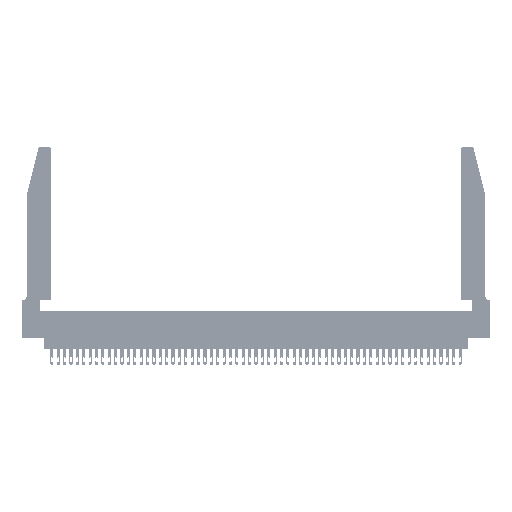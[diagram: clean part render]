
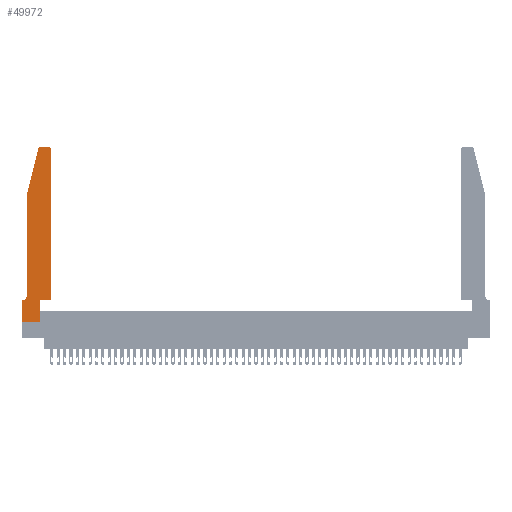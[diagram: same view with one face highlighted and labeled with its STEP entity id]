
A CAD part, top view. The second image highlights one B-rep face of the part: STEP entity #49972.
In plain terms, the highlighted planar face has unit normal (0, 0, 1).
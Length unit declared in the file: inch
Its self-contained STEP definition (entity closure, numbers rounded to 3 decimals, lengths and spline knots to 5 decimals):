
#462 = DIRECTION ( 'NONE',  ( 0., 0., 1. ) ) ;
#658 = CARTESIAN_POINT ( 'NONE',  ( 0.0755, 2., 0.37 ) ) ;
#903 = VERTEX_POINT ( 'NONE', #42194 ) ;
#2040 = CARTESIAN_POINT ( 'NONE',  ( 0.284, 2.75, 0.37 ) ) ;
#2953 = VERTEX_POINT ( 'NONE', #20163 ) ;
#4438 = CARTESIAN_POINT ( 'NONE',  ( 0.0055, 0.42, 0.37 ) ) ;
#5208 = CARTESIAN_POINT ( 'NONE',  ( 0., 0., 0.37 ) ) ;
#5640 = ORIENTED_EDGE ( 'NONE', *, *, #29134, .T. ) ;
#6308 = LINE ( 'NONE', #21184, #25427 ) ;
#6804 = CARTESIAN_POINT ( 'NONE',  ( 0., 0., 0.37 ) ) ;
#7109 = VERTEX_POINT ( 'NONE', #13375 ) ;
#8447 = ORIENTED_EDGE ( 'NONE', *, *, #38276, .T. ) ;
#8705 = DIRECTION ( 'NONE',  ( 1., 0., 0. ) ) ;
#8990 = DIRECTION ( 'NONE',  ( 1., 0., 0. ) ) ;
#9682 = CARTESIAN_POINT ( 'NONE',  ( 0., 0., 0.37 ) ) ;
#9719 = CIRCLE ( 'NONE', #34221, 0.07 ) ;
#10362 = EDGE_CURVE ( 'NONE', #13589, #39218, #52723, .T. ) ;
#10477 = ORIENTED_EDGE ( 'NONE', *, *, #38876, .T. ) ;
#10896 = EDGE_LOOP ( 'NONE', ( #40590, #37836, #21399, #5640, #10477, #12470, #46249, #42510, #8447, #43906, #12363, #19804 ) ) ;
#11210 = VECTOR ( 'NONE', #14097, 39.37008 ) ;
#11883 = EDGE_CURVE ( 'NONE', #49871, #12930, #48112, .T. ) ;
#12033 = CARTESIAN_POINT ( 'NONE',  ( 0.4505, 0.35, 0.37 ) ) ;
#12363 = ORIENTED_EDGE ( 'NONE', *, *, #52319, .T. ) ;
#12470 = ORIENTED_EDGE ( 'NONE', *, *, #20970, .T. ) ;
#12533 = CARTESIAN_POINT ( 'NONE',  ( 0.2865, 0.35, 0.37 ) ) ;
#12930 = VERTEX_POINT ( 'NONE', #16961 ) ;
#13375 = CARTESIAN_POINT ( 'NONE',  ( 0.0055, 0.35, 0.37 ) ) ;
#13589 = VERTEX_POINT ( 'NONE', #49819 ) ;
#14097 = DIRECTION ( 'NONE',  ( 1., 0., 0. ) ) ;
#14239 = LINE ( 'NONE', #9682, #48590 ) ;
#15106 = VECTOR ( 'NONE', #32308, 39.37008 ) ;
#15111 = AXIS2_PLACEMENT_3D ( 'NONE', #41087, #36807, #8705 ) ;
#15677 = DIRECTION ( 'NONE',  ( -1., 0., 0. ) ) ;
#15929 = EDGE_CURVE ( 'NONE', #2953, #44714, #44514, .T. ) ;
#16375 = LINE ( 'NONE', #12033, #15106 ) ;
#16961 = CARTESIAN_POINT ( 'NONE',  ( 0.4505, 0.35, 0.37 ) ) ;
#17741 = CARTESIAN_POINT ( 'NONE',  ( 0.2865, 0., 0.37 ) ) ;
#18474 = EDGE_CURVE ( 'NONE', #903, #32754, #14239, .T. ) ;
#18583 = CIRCLE ( 'NONE', #51100, 0.03 ) ;
#18783 = EDGE_CURVE ( 'NONE', #39218, #41170, #47335, .T. ) ;
#19001 = CARTESIAN_POINT ( 'NONE',  ( 0.4205, 2.75, 0.37 ) ) ;
#19692 = EDGE_CURVE ( 'NONE', #41170, #2953, #18583, .T. ) ;
#19804 = ORIENTED_EDGE ( 'NONE', *, *, #10362, .T. ) ;
#19895 = CARTESIAN_POINT ( 'NONE',  ( 0.2865, 0.35, 0.37 ) ) ;
#20163 = CARTESIAN_POINT ( 'NONE',  ( 0.25487, 2.72718, 0.37 ) ) ;
#20822 = DIRECTION ( 'NONE',  ( -1., 0., 0. ) ) ;
#20970 = EDGE_CURVE ( 'NONE', #7109, #903, #6308, .T. ) ;
#21184 = CARTESIAN_POINT ( 'NONE',  ( 0.0755, 0.35, 0.37 ) ) ;
#21399 = ORIENTED_EDGE ( 'NONE', *, *, #15929, .T. ) ;
#21459 = CARTESIAN_POINT ( 'NONE',  ( 0.0755, 2., 0.37 ) ) ;
#22464 = VECTOR ( 'NONE', #48908, 39.37008 ) ;
#23045 = VECTOR ( 'NONE', #29049, 39.37008 ) ;
#23786 = CARTESIAN_POINT ( 'NONE',  ( 0.0755, 2., 0.37 ) ) ;
#24588 = VERTEX_POINT ( 'NONE', #47378 ) ;
#25427 = VECTOR ( 'NONE', #41481, 39.37008 ) ;
#25846 = DIRECTION ( 'NONE',  ( 0., -1., 0. ) ) ;
#26544 = CARTESIAN_POINT ( 'NONE',  ( 0.284, 2.72, 0.37 ) ) ;
#27489 = LINE ( 'NONE', #12533, #23045 ) ;
#29049 = DIRECTION ( 'NONE',  ( 0., 1., 0. ) ) ;
#29134 = EDGE_CURVE ( 'NONE', #44714, #24588, #38420, .T. ) ;
#29282 = FACE_OUTER_BOUND ( 'NONE', #10896, .T. ) ;
#31175 = CARTESIAN_POINT ( 'NONE',  ( 0.2605, 2.75, 0.37 ) ) ;
#32308 = DIRECTION ( 'NONE',  ( 0., 1., 0. ) ) ;
#32522 = VECTOR ( 'NONE', #8990, 39.37008 ) ;
#32754 = VERTEX_POINT ( 'NONE', #6804 ) ;
#32894 = PLANE ( 'NONE',  #15111 ) ;
#33052 = DIRECTION ( 'NONE',  ( 1., 0., 0. ) ) ;
#34221 = AXIS2_PLACEMENT_3D ( 'NONE', #4438, #41127, #20822 ) ;
#36807 = DIRECTION ( 'NONE',  ( 0., 0., 1. ) ) ;
#36987 = LINE ( 'NONE', #5208, #32522 ) ;
#37033 = CARTESIAN_POINT ( 'NONE',  ( 0.4205, 2.72, 0.37 ) ) ;
#37836 = ORIENTED_EDGE ( 'NONE', *, *, #19692, .T. ) ;
#38276 = EDGE_CURVE ( 'NONE', #50341, #49871, #27489, .T. ) ;
#38420 = LINE ( 'NONE', #658, #22464 ) ;
#38485 = CARTESIAN_POINT ( 'NONE',  ( 0.4505, 0.35, 0.37 ) ) ;
#38876 = EDGE_CURVE ( 'NONE', #24588, #7109, #9719, .T. ) ;
#39218 = VERTEX_POINT ( 'NONE', #19001 ) ;
#39708 = EDGE_CURVE ( 'NONE', #32754, #50341, #36987, .T. ) ;
#40590 = ORIENTED_EDGE ( 'NONE', *, *, #18783, .T. ) ;
#41087 = CARTESIAN_POINT ( 'NONE',  ( 0., 0.35, 0.37 ) ) ;
#41127 = DIRECTION ( 'NONE',  ( 0., 0., -1. ) ) ;
#41170 = VERTEX_POINT ( 'NONE', #2040 ) ;
#41302 = DIRECTION ( 'NONE',  ( 0., 0., 1. ) ) ;
#41481 = DIRECTION ( 'NONE',  ( -1., 0., 0. ) ) ;
#42194 = CARTESIAN_POINT ( 'NONE',  ( 0., 0.35, 0.37 ) ) ;
#42510 = ORIENTED_EDGE ( 'NONE', *, *, #39708, .T. ) ;
#43906 = ORIENTED_EDGE ( 'NONE', *, *, #11883, .T. ) ;
#44514 = LINE ( 'NONE', #21459, #52178 ) ;
#44714 = VERTEX_POINT ( 'NONE', #23786 ) ;
#45031 = DIRECTION ( 'NONE',  ( 1., 0., 0. ) ) ;
#45478 = DIRECTION ( 'NONE',  ( -0.239, -0.971, 0. ) ) ;
#46058 = VECTOR ( 'NONE', #15677, 39.37008 ) ;
#46249 = ORIENTED_EDGE ( 'NONE', *, *, #18474, .T. ) ;
#47335 = LINE ( 'NONE', #31175, #46058 ) ;
#47378 = CARTESIAN_POINT ( 'NONE',  ( 0.0755, 0.42, 0.37 ) ) ;
#48112 = LINE ( 'NONE', #38485, #11210 ) ;
#48590 = VECTOR ( 'NONE', #25846, 39.37008 ) ;
#48908 = DIRECTION ( 'NONE',  ( 0., -1., 0. ) ) ;
#49819 = CARTESIAN_POINT ( 'NONE',  ( 0.4505, 2.72, 0.37 ) ) ;
#49871 = VERTEX_POINT ( 'NONE', #19895 ) ;
#49972 = ADVANCED_FACE ( 'NONE', ( #29282 ), #32894, .T. ) ;
#50341 = VERTEX_POINT ( 'NONE', #17741 ) ;
#51100 = AXIS2_PLACEMENT_3D ( 'NONE', #26544, #462, #33052 ) ;
#51650 = AXIS2_PLACEMENT_3D ( 'NONE', #37033, #41302, #45031 ) ;
#52178 = VECTOR ( 'NONE', #45478, 39.37008 ) ;
#52319 = EDGE_CURVE ( 'NONE', #12930, #13589, #16375, .T. ) ;
#52723 = CIRCLE ( 'NONE', #51650, 0.03 ) ;
